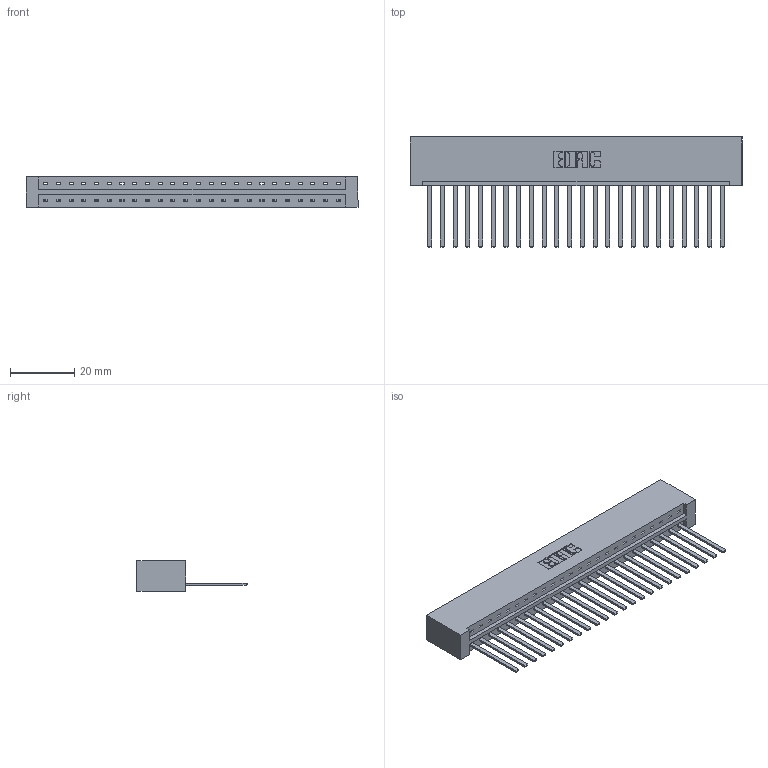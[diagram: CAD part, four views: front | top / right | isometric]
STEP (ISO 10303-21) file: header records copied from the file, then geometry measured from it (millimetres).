
FILE_DESCRIPTION (( 'STEP AP203' ), '1' );
FILE_NAME ('833-024-544-101.STEP', '2020-06-01T21:50:05', ( '' ), ( '' ), 'SwSTEP 2.0', 'SolidWorks 2020', '' );
FILE_SCHEMA (( 'CONFIG_CONTROL_DESIGN' ));
Length unit declared in the file: inch
Products named in the file (3): 345-292-001_345-293-144; 833 Part_Lugless; 833-024-544-101
Assembly tree (25 placements, depth 2):
  833-024-544-101
    833 Part_Lugless
    345-292-001_345-293-144  x24
Bounding box: 103.35 x 34.3 x 9.4 mm (x, y, z)
Volume: 11136.1 mm3; surface area: 12791.6 mm2
Topology: 25 solids, 25 shells, 1354 faces, 4079 edges, 2686 vertices
Faces by surface type: plane 978, cylinder 376
Entity records: 16539 total; most frequent: CARTESIAN_POINT 2862, ORIENTED_EDGE 2822, DIRECTION 2439, EDGE_CURVE 1411, VECTOR 1295, LINE 1295, VERTEX_POINT 938, AXIS2_PLACEMENT_3D 572
